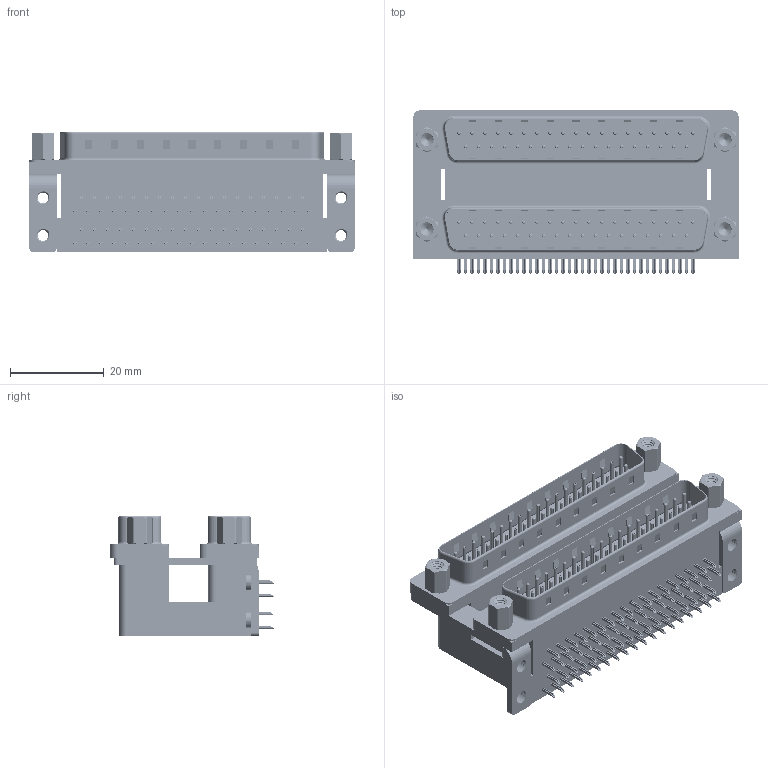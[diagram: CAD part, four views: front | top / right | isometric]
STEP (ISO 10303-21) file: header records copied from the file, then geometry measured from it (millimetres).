
FILE_DESCRIPTION (( 'STEP AP203' ), '1' );
FILE_NAME ('661-037-264-056.STEP', '2022-06-15T21:45:28', ( '' ), ( '' ), 'SwSTEP 2.0', 'SolidWorks 2020', '' );
FILE_SCHEMA (( 'CONFIG_CONTROL_DESIGN' ));
Length unit declared in the file: millimetre
Products named in the file (13): 661 Contact Top Upper_M; 661 Mounting Bracket_ThruM; 661 Shell_37 Contacts; 661 Contact Top Lower; 661 Housing Lower_37 Contacts; 661 4-40 Hex Standoff 5; 661 4-40 Threaded Board Mount; 661 Contact Bottom Upper_M; 661 Contact Bottom Lower; 661-037-264-056; 661 Threaded Rivet_4-40; 661 Housing Upper_37 Contacts M; 661 Housing Spacer_37 Contacts M
Assembly tree (93 placements, depth 2):
  661-037-264-056
    661 Housing Lower_37 Contacts
    661 Housing Spacer_37 Contacts M
    661 Housing Upper_37 Contacts M
    661 Shell_37 Contacts  x2
    661 Contact Bottom Lower  x18
    661 Contact Top Lower  x19
    661 Contact Bottom Upper_M  x18
    661 Contact Top Upper_M  x19
    661 Mounting Bracket_ThruM  x2
    661 4-40 Threaded Board Mount  x4
    661 Threaded Rivet_4-40  x4
    661 4-40 Hex Standoff 5  x4
Bounding box: 69.32 x 34.78 x 25.6 mm (x, y, z)
Volume: 29711.1 mm3; surface area: 30977.2 mm2
Topology: 93 solids, 93 shells, 6974 faces, 17372 edges, 10762 vertices
Faces by surface type: plane 4306, cylinder 2014, torus 506, cone 100, bspline 48
Entity records: 57958 total; most frequent: CARTESIAN_POINT 14457, ORIENTED_EDGE 8164, DIRECTION 8138, EDGE_CURVE 4082, VECTOR 3080, LINE 3080, VERTEX_POINT 2651, AXIS2_PLACEMENT_3D 2529
